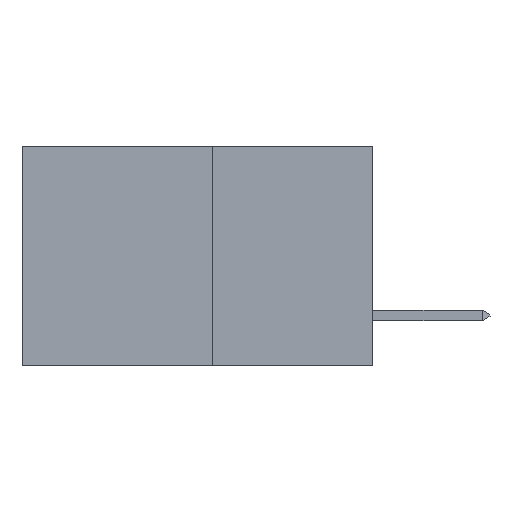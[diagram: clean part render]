
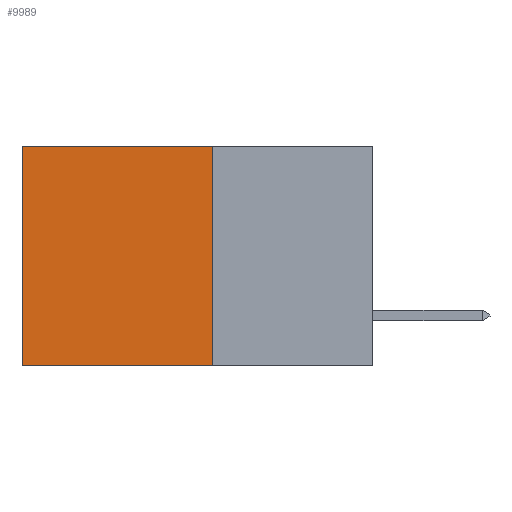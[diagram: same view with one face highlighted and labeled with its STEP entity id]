
A CAD part, left-side view. The second image highlights one B-rep face of the part: STEP entity #9989.
In plain terms, the highlighted planar face has unit normal (-1, 0, 0).
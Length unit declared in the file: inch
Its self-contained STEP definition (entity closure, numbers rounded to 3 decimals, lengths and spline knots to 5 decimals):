
#322 = LINE ( 'NONE', #1273, #2456 ) ;
#438 = EDGE_CURVE ( 'NONE', #2775, #6866, #472, .T. ) ;
#472 = LINE ( 'NONE', #7070, #2043 ) ;
#619 = EDGE_CURVE ( 'NONE', #7650, #5517, #322, .T. ) ;
#664 = ORIENTED_EDGE ( 'NONE', *, *, #438, .F. ) ;
#1220 = CARTESIAN_POINT ( 'NONE',  ( 0.277, 0.27, -0.37 ) ) ;
#1273 = CARTESIAN_POINT ( 'NONE',  ( 0.277, 0.27, 0. ) ) ;
#1660 = DIRECTION ( 'NONE',  ( 0., 1., 0. ) ) ;
#1828 = ORIENTED_EDGE ( 'NONE', *, *, #619, .T. ) ;
#2043 = VECTOR ( 'NONE', #7367, 39.37008 ) ;
#2195 = PLANE ( 'NONE',  #7498 ) ;
#2343 = CARTESIAN_POINT ( 'NONE',  ( 0.277, 0.27, -0.37 ) ) ;
#2456 = VECTOR ( 'NONE', #1660, 39.37008 ) ;
#2775 = VERTEX_POINT ( 'NONE', #2343 ) ;
#3068 = CARTESIAN_POINT ( 'NONE',  ( 0.277, 0.59, 0. ) ) ;
#3450 = ORIENTED_EDGE ( 'NONE', *, *, #6961, .F. ) ;
#4031 = DIRECTION ( 'NONE',  ( 0., 0., -1. ) ) ;
#4034 = VECTOR ( 'NONE', #8517, 39.37008 ) ;
#4404 = EDGE_CURVE ( 'NONE', #5517, #6866, #11276, .T. ) ;
#4711 = LINE ( 'NONE', #9728, #6861 ) ;
#5517 = VERTEX_POINT ( 'NONE', #3068 ) ;
#5937 = CARTESIAN_POINT ( 'NONE',  ( 0.277, 0.59, -0.37 ) ) ;
#6157 = EDGE_LOOP ( 'NONE', ( #10824, #664, #3450, #1828 ) ) ;
#6861 = VECTOR ( 'NONE', #10609, 39.37008 ) ;
#6866 = VERTEX_POINT ( 'NONE', #5937 ) ;
#6961 = EDGE_CURVE ( 'NONE', #7650, #2775, #4711, .T. ) ;
#7070 = CARTESIAN_POINT ( 'NONE',  ( 0.277, 0.27, -0.37 ) ) ;
#7367 = DIRECTION ( 'NONE',  ( 0., 1., 0. ) ) ;
#7498 = AXIS2_PLACEMENT_3D ( 'NONE', #1220, #9490, #4031 ) ;
#7650 = VERTEX_POINT ( 'NONE', #11526 ) ;
#8517 = DIRECTION ( 'NONE',  ( 0., 0., -1. ) ) ;
#8746 = FACE_OUTER_BOUND ( 'NONE', #6157, .T. ) ;
#9490 = DIRECTION ( 'NONE',  ( 1., 0., 0. ) ) ;
#9728 = CARTESIAN_POINT ( 'NONE',  ( 0.277, 0.27, -0.37 ) ) ;
#9989 = ADVANCED_FACE ( 'NONE', ( #8746 ), #2195, .F. ) ;
#10017 = CARTESIAN_POINT ( 'NONE',  ( 0.277, 0.59, -0.37 ) ) ;
#10609 = DIRECTION ( 'NONE',  ( 0., 0., -1. ) ) ;
#10824 = ORIENTED_EDGE ( 'NONE', *, *, #4404, .T. ) ;
#11276 = LINE ( 'NONE', #10017, #4034 ) ;
#11526 = CARTESIAN_POINT ( 'NONE',  ( 0.277, 0.27, 0. ) ) ;
